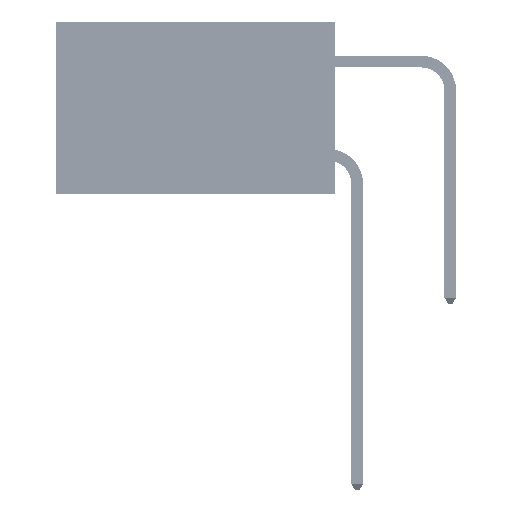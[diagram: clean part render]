
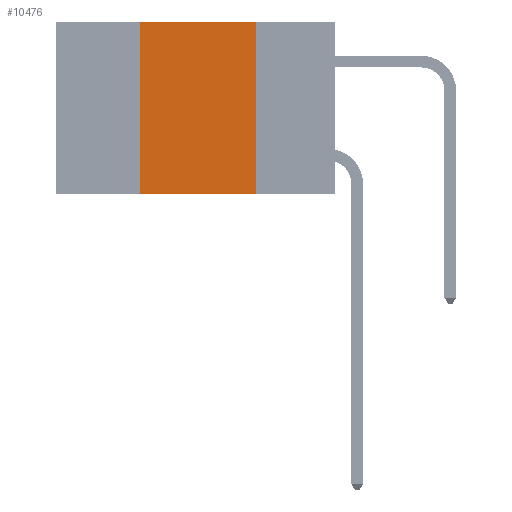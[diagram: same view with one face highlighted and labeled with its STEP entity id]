
A CAD part, left-side view. The second image highlights one B-rep face of the part: STEP entity #10476.
In plain terms, the highlighted planar face has unit normal (-1, 0, 0).
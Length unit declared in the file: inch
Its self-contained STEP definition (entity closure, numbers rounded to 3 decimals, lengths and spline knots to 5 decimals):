
#357 = VERTEX_POINT ( 'NONE', #24075 ) ;
#735 = ORIENTED_EDGE ( 'NONE', *, *, #9520, .F. ) ;
#1278 = CARTESIAN_POINT ( 'NONE',  ( 0., 0.17, 0. ) ) ;
#3130 = CARTESIAN_POINT ( 'NONE',  ( 0., 0.42, 0. ) ) ;
#4817 = VECTOR ( 'NONE', #14518, 39.37008 ) ;
#5847 = LINE ( 'NONE', #26208, #14011 ) ;
#6995 = CARTESIAN_POINT ( 'NONE',  ( 0., 0.17, 0. ) ) ;
#9520 = EDGE_CURVE ( 'NONE', #37305, #41169, #48070, .T. ) ;
#10476 = ADVANCED_FACE ( 'NONE', ( #47386 ), #39281, .F. ) ;
#12582 = ORIENTED_EDGE ( 'NONE', *, *, #31855, .F. ) ;
#14011 = VECTOR ( 'NONE', #15853, 39.37008 ) ;
#14518 = DIRECTION ( 'NONE',  ( 0., 0., 1. ) ) ;
#14817 = DIRECTION ( 'NONE',  ( 0., 0., -1. ) ) ;
#15830 = VECTOR ( 'NONE', #34226, 39.37008 ) ;
#15853 = DIRECTION ( 'NONE',  ( 0., -1., 0. ) ) ;
#18184 = EDGE_CURVE ( 'NONE', #37305, #357, #5847, .T. ) ;
#20636 = CARTESIAN_POINT ( 'NONE',  ( 0., 0.6, 0. ) ) ;
#21526 = AXIS2_PLACEMENT_3D ( 'NONE', #20636, #46784, #37142 ) ;
#21748 = ORIENTED_EDGE ( 'NONE', *, *, #18184, .T. ) ;
#24075 = CARTESIAN_POINT ( 'NONE',  ( 0., 0.17, -0.37 ) ) ;
#24675 = LINE ( 'NONE', #30492, #15830 ) ;
#25037 = LINE ( 'NONE', #6995, #40831 ) ;
#26208 = CARTESIAN_POINT ( 'NONE',  ( 0., 0.6, -0.37 ) ) ;
#28729 = CARTESIAN_POINT ( 'NONE',  ( 0., 0.42, -0.37 ) ) ;
#30492 = CARTESIAN_POINT ( 'NONE',  ( 0., 0.6, 0. ) ) ;
#31560 = ORIENTED_EDGE ( 'NONE', *, *, #35887, .F. ) ;
#31855 = EDGE_CURVE ( 'NONE', #41169, #45984, #24675, .T. ) ;
#34226 = DIRECTION ( 'NONE',  ( 0., -1., 0. ) ) ;
#35055 = CARTESIAN_POINT ( 'NONE',  ( 0., 0.42, 0. ) ) ;
#35887 = EDGE_CURVE ( 'NONE', #45984, #357, #25037, .T. ) ;
#37142 = DIRECTION ( 'NONE',  ( 0., 0., -1. ) ) ;
#37305 = VERTEX_POINT ( 'NONE', #28729 ) ;
#39281 = PLANE ( 'NONE',  #21526 ) ;
#40831 = VECTOR ( 'NONE', #14817, 39.37008 ) ;
#41169 = VERTEX_POINT ( 'NONE', #35055 ) ;
#45984 = VERTEX_POINT ( 'NONE', #1278 ) ;
#46784 = DIRECTION ( 'NONE',  ( 1., 0., 0. ) ) ;
#47386 = FACE_OUTER_BOUND ( 'NONE', #48071, .T. ) ;
#48070 = LINE ( 'NONE', #3130, #4817 ) ;
#48071 = EDGE_LOOP ( 'NONE', ( #31560, #12582, #735, #21748 ) ) ;
